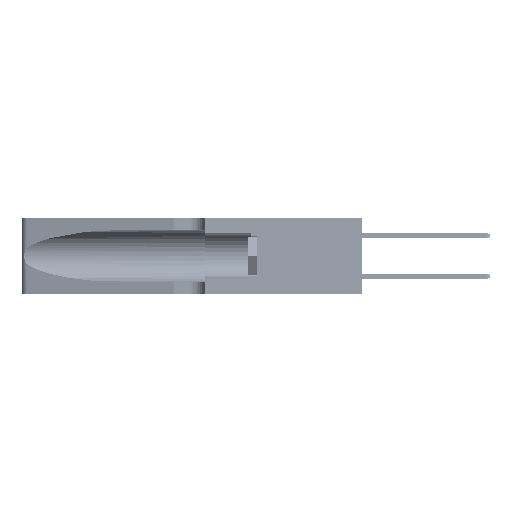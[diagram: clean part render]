
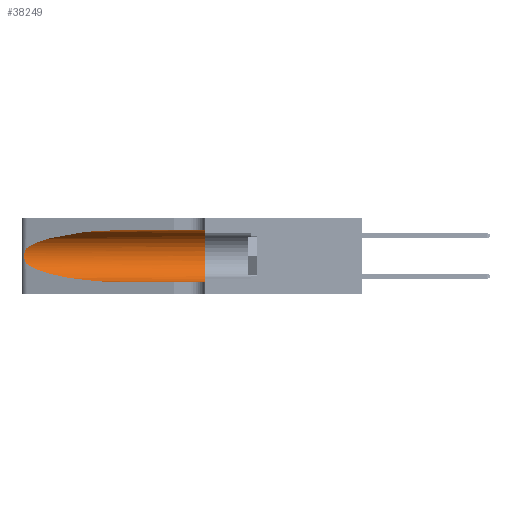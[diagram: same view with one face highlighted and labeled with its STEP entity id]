
A CAD part, left-side view. The second image highlights one B-rep face of the part: STEP entity #38249.
In plain terms, the highlighted cylindrical face has radius 3.308 mm (diameter 6.617 mm), a partial arc.
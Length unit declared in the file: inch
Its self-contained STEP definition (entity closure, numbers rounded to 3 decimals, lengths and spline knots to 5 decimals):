
#20 = CARTESIAN_POINT ( 'NONE',  ( 0.18966, 0.96281, 0.31525 ) ) ;
#1512 = EDGE_CURVE ( 'NONE', #12958, #30682, #46421, .T. ) ;
#2276 = CARTESIAN_POINT ( 'NONE',  ( 0.25555, 1.22994, 0.2215 ) ) ;
#3956 = CARTESIAN_POINT ( 'NONE',  ( 0.1305, 0.72297, 0.31525 ) ) ;
#4671 = CARTESIAN_POINT ( 'NONE',  ( 0.2373, 1.15595, 0.08982 ) ) ;
#4674 = B_SPLINE_CURVE_WITH_KNOTS ( 'NONE', 3,
 ( #48734, #2276, #29591, #6209, #33483, #10131, #37319, #14047, #41192, #17996, #45055, #21918, #48915, #25866 ),
 .UNSPECIFIED., .F., .F.,
 ( 4, 2, 2, 2, 2, 2, 4 ),
 ( 0., 0.00027, 0.00053, 0.00107, 0.0016, 0.00187, 0.00214 ),
 .UNSPECIFIED. ) ;
#5692 = DIRECTION ( 'NONE',  ( 0., 0., -1. ) ) ;
#6209 = CARTESIAN_POINT ( 'NONE',  ( 0.25787, 1.23484, 0.2124 ) ) ;
#6372 = EDGE_CURVE ( 'NONE', #46663, #27091, #10006, .T. ) ;
#6715 = CARTESIAN_POINT ( 'NONE',  ( 0.1305, 0.35, 0.31525 ) ) ;
#6832 = CARTESIAN_POINT ( 'NONE',  ( 0.1305, 0.72297, 0.05475 ) ) ;
#7911 = CARTESIAN_POINT ( 'NONE',  ( 0.25487, 1.22718, 0.22369 ) ) ;
#9622 = DIRECTION ( 'NONE',  ( 0., -1., 0. ) ) ;
#9981 = ORIENTED_EDGE ( 'NONE', *, *, #38769, .F. ) ;
#10006 =( BOUNDED_CURVE ( )  B_SPLINE_CURVE ( 3, ( #3956, #20, #23441, #7911 ),
 .UNSPECIFIED., .F., .T. ) 
 B_SPLINE_CURVE_WITH_KNOTS ( ( 4, 4 ),
 ( 1.5708, 2.84003 ),
 .UNSPECIFIED. ) 
 CURVE ( )  GEOMETRIC_REPRESENTATION_ITEM ( )  RATIONAL_B_SPLINE_CURVE ( ( 1., 0.87, 0.87, 1. ) ) 
 REPRESENTATION_ITEM ( '' )  );
#10131 = CARTESIAN_POINT ( 'NONE',  ( 0.26018, 1.23835, 0.19895 ) ) ;
#10519 = LINE ( 'NONE', #47840, #49302 ) ;
#12212 = EDGE_CURVE ( 'NONE', #27091, #14988, #4674, .T. ) ;
#12537 = CARTESIAN_POINT ( 'NONE',  ( 0.18966, 0.96281, 0.05475 ) ) ;
#12958 = VERTEX_POINT ( 'NONE', #6832 ) ;
#12987 = EDGE_LOOP ( 'NONE', ( #43116, #36497, #16948, #38396, #14083, #9981 ) ) ;
#13022 = FACE_OUTER_BOUND ( 'NONE', #12987, .T. ) ;
#14047 = CARTESIAN_POINT ( 'NONE',  ( 0.26075, 1.23896, 0.178 ) ) ;
#14083 = ORIENTED_EDGE ( 'NONE', *, *, #40888, .F. ) ;
#14242 = CYLINDRICAL_SURFACE ( 'NONE', #25917, 0.13025 ) ;
#14988 = VERTEX_POINT ( 'NONE', #34913 ) ;
#16889 =( BOUNDED_CURVE ( )  B_SPLINE_CURVE ( 3, ( #31970, #4671, #12537, #39671 ),
 .UNSPECIFIED., .F., .T. ) 
 B_SPLINE_CURVE_WITH_KNOTS ( ( 4, 4 ),
 ( 3.44316, 4.71239 ),
 .UNSPECIFIED. ) 
 CURVE ( )  GEOMETRIC_REPRESENTATION_ITEM ( )  RATIONAL_B_SPLINE_CURVE ( ( 1., 0.87, 0.87, 1. ) ) 
 REPRESENTATION_ITEM ( '' )  );
#16948 = ORIENTED_EDGE ( 'NONE', *, *, #49146, .T. ) ;
#17333 = CARTESIAN_POINT ( 'NONE',  ( 0.1305, 0.35, 0.185 ) ) ;
#17996 = CARTESIAN_POINT ( 'NONE',  ( 0.25856, 1.23593, 0.16098 ) ) ;
#21261 = DIRECTION ( 'NONE',  ( 0., 0., 1. ) ) ;
#21918 = CARTESIAN_POINT ( 'NONE',  ( 0.25639, 1.23186, 0.15144 ) ) ;
#23441 = CARTESIAN_POINT ( 'NONE',  ( 0.2373, 1.15595, 0.28018 ) ) ;
#25866 = CARTESIAN_POINT ( 'NONE',  ( 0.25487, 1.22718, 0.14631 ) ) ;
#25917 = AXIS2_PLACEMENT_3D ( 'NONE', #36667, #9622, #5692 ) ;
#27042 = CARTESIAN_POINT ( 'NONE',  ( 0.1305, 0.35, 0.05475 ) ) ;
#27091 = VERTEX_POINT ( 'NONE', #39011 ) ;
#28523 = DIRECTION ( 'NONE',  ( 0., -1., 0. ) ) ;
#29591 = CARTESIAN_POINT ( 'NONE',  ( 0.25639, 1.23184, 0.21858 ) ) ;
#30682 = VERTEX_POINT ( 'NONE', #27042 ) ;
#31970 = CARTESIAN_POINT ( 'NONE',  ( 0.25487, 1.22718, 0.14631 ) ) ;
#33483 = CARTESIAN_POINT ( 'NONE',  ( 0.25854, 1.2359, 0.20912 ) ) ;
#34913 = CARTESIAN_POINT ( 'NONE',  ( 0.25487, 1.22718, 0.14631 ) ) ;
#36013 = VERTEX_POINT ( 'NONE', #6715 ) ;
#36497 = ORIENTED_EDGE ( 'NONE', *, *, #12212, .T. ) ;
#36667 = CARTESIAN_POINT ( 'NONE',  ( 0.1305, 1.61858, 0.185 ) ) ;
#37319 = CARTESIAN_POINT ( 'NONE',  ( 0.26075, 1.23896, 0.19203 ) ) ;
#38249 = ADVANCED_FACE ( 'NONE', ( #13022 ), #14242, .F. ) ;
#38396 = ORIENTED_EDGE ( 'NONE', *, *, #1512, .T. ) ;
#38769 = EDGE_CURVE ( 'NONE', #46663, #36013, #10519, .T. ) ;
#39011 = CARTESIAN_POINT ( 'NONE',  ( 0.25487, 1.22718, 0.22369 ) ) ;
#39671 = CARTESIAN_POINT ( 'NONE',  ( 0.1305, 0.72297, 0.05475 ) ) ;
#40888 = EDGE_CURVE ( 'NONE', #36013, #30682, #44363, .T. ) ;
#41192 = CARTESIAN_POINT ( 'NONE',  ( 0.26017, 1.23833, 0.17102 ) ) ;
#43116 = ORIENTED_EDGE ( 'NONE', *, *, #6372, .T. ) ;
#44037 = CARTESIAN_POINT ( 'NONE',  ( 0.1305, 0.72297, 0.31525 ) ) ;
#44363 = CIRCLE ( 'NONE', #45709, 0.13025 ) ;
#44415 = DIRECTION ( 'NONE',  ( 0., 1., 0. ) ) ;
#45055 = CARTESIAN_POINT ( 'NONE',  ( 0.25789, 1.23486, 0.15765 ) ) ;
#45212 = VECTOR ( 'NONE', #49746, 39.37008 ) ;
#45709 = AXIS2_PLACEMENT_3D ( 'NONE', #17333, #44415, #21261 ) ;
#45892 = CARTESIAN_POINT ( 'NONE',  ( 0.1305, 1.61858, 0.05475 ) ) ;
#46421 = LINE ( 'NONE', #45892, #45212 ) ;
#46663 = VERTEX_POINT ( 'NONE', #44037 ) ;
#47840 = CARTESIAN_POINT ( 'NONE',  ( 0.1305, 1.61858, 0.31525 ) ) ;
#48734 = CARTESIAN_POINT ( 'NONE',  ( 0.25487, 1.22718, 0.22369 ) ) ;
#48915 = CARTESIAN_POINT ( 'NONE',  ( 0.25555, 1.22993, 0.14849 ) ) ;
#49146 = EDGE_CURVE ( 'NONE', #14988, #12958, #16889, .T. ) ;
#49302 = VECTOR ( 'NONE', #28523, 39.37008 ) ;
#49746 = DIRECTION ( 'NONE',  ( 0., -1., 0. ) ) ;
